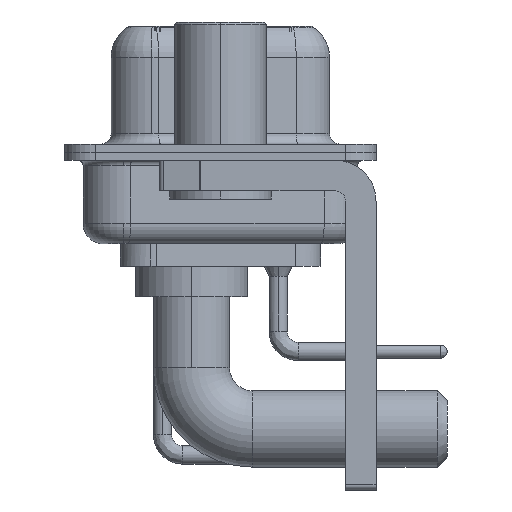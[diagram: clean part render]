
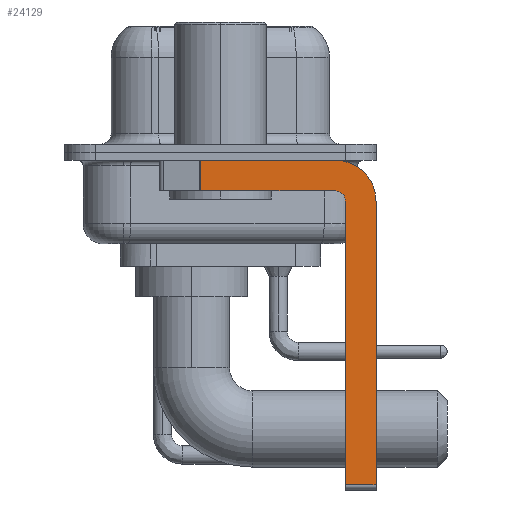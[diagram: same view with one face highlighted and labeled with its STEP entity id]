
A CAD part, left-side view. The second image highlights one B-rep face of the part: STEP entity #24129.
In plain terms, the highlighted planar face has unit normal (-1, 0, 0).
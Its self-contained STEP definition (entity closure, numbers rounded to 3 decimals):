
#1060 = DIRECTION ( 'NONE',  ( 0., 0., 1. ) ) ;
#1288 = CARTESIAN_POINT ( 'NONE',  ( -2.9, 0.978, -1.9 ) ) ;
#1425 = ORIENTED_EDGE ( 'NONE', *, *, #20776, .F. ) ;
#2967 = PLANE ( 'NONE',  #27214 ) ;
#3376 = DIRECTION ( 'NONE',  ( 0., -1., 0. ) ) ;
#3936 = VERTEX_POINT ( 'NONE', #34756 ) ;
#3948 = VECTOR ( 'NONE', #10838, 1000. ) ;
#5641 = ORIENTED_EDGE ( 'NONE', *, *, #31701, .F. ) ;
#5891 = CIRCLE ( 'NONE', #11822, 0.5 ) ;
#5926 = CIRCLE ( 'NONE', #10030, 2. ) ;
#6076 = VECTOR ( 'NONE', #19685, 1000. ) ;
#6174 = ORIENTED_EDGE ( 'NONE', *, *, #34857, .T. ) ;
#7104 = VECTOR ( 'NONE', #3376, 1000. ) ;
#7942 = EDGE_LOOP ( 'NONE', ( #22474, #6174, #32761, #15115, #1425, #31337, #5641, #16504 ) ) ;
#8056 = LINE ( 'NONE', #35947, #6076 ) ;
#8319 = FACE_OUTER_BOUND ( 'NONE', #7942, .T. ) ;
#10030 = AXIS2_PLACEMENT_3D ( 'NONE', #14825, #34590, #17969 ) ;
#10592 = DIRECTION ( 'NONE',  ( -1., 0., 0. ) ) ;
#10838 = DIRECTION ( 'NONE',  ( 0., 0., 1. ) ) ;
#11681 = LINE ( 'NONE', #29431, #7104 ) ;
#11822 = AXIS2_PLACEMENT_3D ( 'NONE', #20812, #10592, #1060 ) ;
#13978 = VERTEX_POINT ( 'NONE', #19483 ) ;
#14825 = CARTESIAN_POINT ( 'NONE',  ( -2.9, -5.65, -2.4 ) ) ;
#15100 = VERTEX_POINT ( 'NONE', #1288 ) ;
#15115 = ORIENTED_EDGE ( 'NONE', *, *, #24831, .F. ) ;
#15508 = DIRECTION ( 'NONE',  ( 0., 0., -1. ) ) ;
#16342 = VERTEX_POINT ( 'NONE', #19746 ) ;
#16504 = ORIENTED_EDGE ( 'NONE', *, *, #23457, .F. ) ;
#16564 = LINE ( 'NONE', #25062, #3948 ) ;
#17969 = DIRECTION ( 'NONE',  ( 0., 0., -1. ) ) ;
#18280 = LINE ( 'NONE', #24191, #23505 ) ;
#18299 = VECTOR ( 'NONE', #32879, 1000. ) ;
#19059 = CARTESIAN_POINT ( 'NONE',  ( -2.9, 0.978, -0.4 ) ) ;
#19406 = CARTESIAN_POINT ( 'NONE',  ( -2.9, -7.65, -2.4 ) ) ;
#19483 = CARTESIAN_POINT ( 'NONE',  ( -2.9, -5.65, -1.9 ) ) ;
#19582 = DIRECTION ( 'NONE',  ( 1., 0., 0. ) ) ;
#19685 = DIRECTION ( 'NONE',  ( 0., 1., 0. ) ) ;
#19746 = CARTESIAN_POINT ( 'NONE',  ( -2.9, -5.65, -0.4 ) ) ;
#19796 = VERTEX_POINT ( 'NONE', #19406 ) ;
#20776 = EDGE_CURVE ( 'NONE', #31923, #3936, #16564, .T. ) ;
#20812 = CARTESIAN_POINT ( 'NONE',  ( -2.9, -5.65, -2.4 ) ) ;
#22474 = ORIENTED_EDGE ( 'NONE', *, *, #25088, .F. ) ;
#22694 = CARTESIAN_POINT ( 'NONE',  ( -2.9, -7.65, -16.35 ) ) ;
#23457 = EDGE_CURVE ( 'NONE', #16342, #19796, #5926, .T. ) ;
#23505 = VECTOR ( 'NONE', #15508, 1000. ) ;
#24129 = ADVANCED_FACE ( 'NONE', ( #8319 ), #2967, .F. ) ;
#24191 = CARTESIAN_POINT ( 'NONE',  ( -2.9, -7.65, -2.4 ) ) ;
#24831 = EDGE_CURVE ( 'NONE', #3936, #13978, #5891, .T. ) ;
#25062 = CARTESIAN_POINT ( 'NONE',  ( -2.9, -6.15, -16.6 ) ) ;
#25088 = EDGE_CURVE ( 'NONE', #33175, #16342, #11681, .T. ) ;
#25489 = VECTOR ( 'NONE', #33538, 1000. ) ;
#26475 = EDGE_CURVE ( 'NONE', #31923, #27300, #36478, .T. ) ;
#27214 = AXIS2_PLACEMENT_3D ( 'NONE', #35842, #19582, #30504 ) ;
#27300 = VERTEX_POINT ( 'NONE', #22694 ) ;
#27529 = CARTESIAN_POINT ( 'NONE',  ( -2.9, 0.978, -1.9 ) ) ;
#27691 = EDGE_CURVE ( 'NONE', #13978, #15100, #8056, .T. ) ;
#27834 = CARTESIAN_POINT ( 'NONE',  ( -2.9, -5.65, -16.35 ) ) ;
#29431 = CARTESIAN_POINT ( 'NONE',  ( -2.9, 3., -0.4 ) ) ;
#30504 = DIRECTION ( 'NONE',  ( 0., 0., -1. ) ) ;
#31337 = ORIENTED_EDGE ( 'NONE', *, *, #26475, .T. ) ;
#31701 = EDGE_CURVE ( 'NONE', #19796, #27300, #18280, .T. ) ;
#31923 = VERTEX_POINT ( 'NONE', #35994 ) ;
#32761 = ORIENTED_EDGE ( 'NONE', *, *, #27691, .F. ) ;
#32879 = DIRECTION ( 'NONE',  ( 0., 0., -1. ) ) ;
#33175 = VERTEX_POINT ( 'NONE', #19059 ) ;
#33538 = DIRECTION ( 'NONE',  ( 0., -1., 0. ) ) ;
#34590 = DIRECTION ( 'NONE',  ( 1., 0., 0. ) ) ;
#34756 = CARTESIAN_POINT ( 'NONE',  ( -2.9, -6.15, -2.4 ) ) ;
#34857 = EDGE_CURVE ( 'NONE', #33175, #15100, #35638, .T. ) ;
#35638 = LINE ( 'NONE', #27529, #18299 ) ;
#35842 = CARTESIAN_POINT ( 'NONE',  ( -2.9, -5.65, -2.4 ) ) ;
#35947 = CARTESIAN_POINT ( 'NONE',  ( -2.9, -5.65, -1.9 ) ) ;
#35994 = CARTESIAN_POINT ( 'NONE',  ( -2.9, -6.15, -16.35 ) ) ;
#36478 = LINE ( 'NONE', #27834, #25489 ) ;
